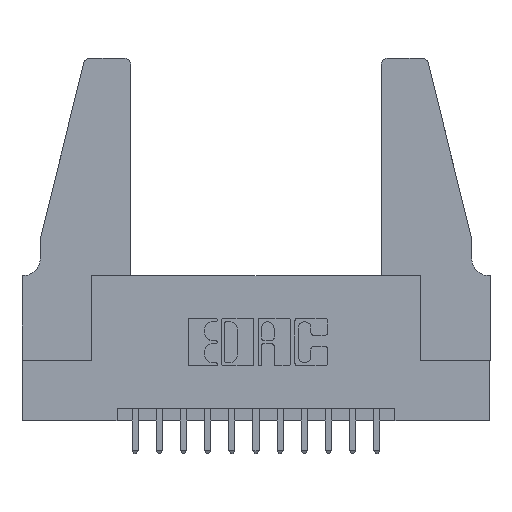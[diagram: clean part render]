
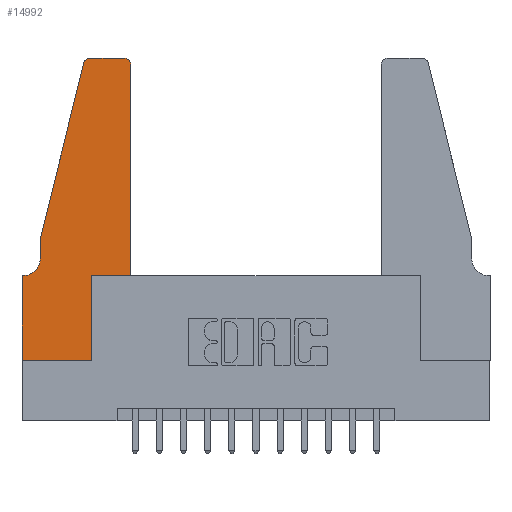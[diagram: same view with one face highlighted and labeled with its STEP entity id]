
A CAD part, top view. The second image highlights one B-rep face of the part: STEP entity #14992.
In plain terms, the highlighted planar face has unit normal (0, 0, 1).
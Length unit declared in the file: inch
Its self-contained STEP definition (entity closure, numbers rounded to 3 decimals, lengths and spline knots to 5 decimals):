
#108 = CARTESIAN_POINT ( 'NONE',  ( 0.0755, 0.5, 0.37 ) ) ;
#125 = VERTEX_POINT ( 'NONE', #3327 ) ;
#166 = DIRECTION ( 'NONE',  ( 0., -1., 0. ) ) ;
#212 = ORIENTED_EDGE ( 'NONE', *, *, #12947, .T. ) ;
#228 = EDGE_CURVE ( 'NONE', #125, #12000, #5634, .T. ) ;
#262 = CARTESIAN_POINT ( 'NONE',  ( 0.0755, 0.5, 0.37 ) ) ;
#379 = LINE ( 'NONE', #500, #3182 ) ;
#433 = CARTESIAN_POINT ( 'NONE',  ( 0.0755, 0.5, 0.37 ) ) ;
#470 = FACE_OUTER_BOUND ( 'NONE', #2129, .T. ) ;
#500 = CARTESIAN_POINT ( 'NONE',  ( 0., 0., 0.37 ) ) ;
#757 = EDGE_CURVE ( 'NONE', #13732, #3302, #10643, .T. ) ;
#803 = CARTESIAN_POINT ( 'NONE',  ( 0.284, 1.22, 0.37 ) ) ;
#858 = CARTESIAN_POINT ( 'NONE',  ( 0.284, 1.25, 0.37 ) ) ;
#1030 = VERTEX_POINT ( 'NONE', #3414 ) ;
#1486 = CIRCLE ( 'NONE', #11365, 0.03 ) ;
#1576 = VERTEX_POINT ( 'NONE', #4155 ) ;
#1954 = CARTESIAN_POINT ( 'NONE',  ( 0.2865, 0.35, 0.37 ) ) ;
#1992 = DIRECTION ( 'NONE',  ( 1., 0., 0. ) ) ;
#2028 = DIRECTION ( 'NONE',  ( 1., 0., 0. ) ) ;
#2129 = EDGE_LOOP ( 'NONE', ( #12750, #11359, #11556, #3574, #4023, #6680, #8276, #8024, #5431, #2158, #8148, #212 ) ) ;
#2158 = ORIENTED_EDGE ( 'NONE', *, *, #7189, .T. ) ;
#2525 = VECTOR ( 'NONE', #5208, 39.37008 ) ;
#2835 = LINE ( 'NONE', #433, #14681 ) ;
#2880 = EDGE_CURVE ( 'NONE', #14587, #1576, #11490, .T. ) ;
#2937 = CARTESIAN_POINT ( 'NONE',  ( 0.4505, 0.35, 0.37 ) ) ;
#2989 = EDGE_CURVE ( 'NONE', #12777, #125, #379, .T. ) ;
#3182 = VECTOR ( 'NONE', #9149, 39.37008 ) ;
#3302 = VERTEX_POINT ( 'NONE', #858 ) ;
#3327 = CARTESIAN_POINT ( 'NONE',  ( 0., 0., 0.37 ) ) ;
#3397 = CARTESIAN_POINT ( 'NONE',  ( 0., 0.35, 0.37 ) ) ;
#3414 = CARTESIAN_POINT ( 'NONE',  ( 0.4505, 1.22, 0.37 ) ) ;
#3507 = EDGE_CURVE ( 'NONE', #14669, #12777, #5528, .T. ) ;
#3574 = ORIENTED_EDGE ( 'NONE', *, *, #2880, .T. ) ;
#3804 = DIRECTION ( 'NONE',  ( 0., 0., -1. ) ) ;
#4023 = ORIENTED_EDGE ( 'NONE', *, *, #7883, .T. ) ;
#4064 = EDGE_CURVE ( 'NONE', #9768, #1030, #13223, .T. ) ;
#4136 = AXIS2_PLACEMENT_3D ( 'NONE', #803, #8943, #1992 ) ;
#4155 = CARTESIAN_POINT ( 'NONE',  ( 0.0755, 0.42, 0.37 ) ) ;
#4530 = VECTOR ( 'NONE', #4562, 39.37008 ) ;
#4562 = DIRECTION ( 'NONE',  ( -1., 0., 0. ) ) ;
#4564 = DIRECTION ( 'NONE',  ( 1., 0., 0. ) ) ;
#4651 = VECTOR ( 'NONE', #166, 39.37008 ) ;
#4653 = CARTESIAN_POINT ( 'NONE',  ( 0.4205, 1.25, 0.37 ) ) ;
#5072 = DIRECTION ( 'NONE',  ( 0., 0., 1. ) ) ;
#5208 = DIRECTION ( 'NONE',  ( 1., 0., 0. ) ) ;
#5271 = DIRECTION ( 'NONE',  ( 0., 1., 0. ) ) ;
#5431 = ORIENTED_EDGE ( 'NONE', *, *, #9946, .T. ) ;
#5528 = LINE ( 'NONE', #5904, #11278 ) ;
#5634 = LINE ( 'NONE', #11948, #2525 ) ;
#5657 = LINE ( 'NONE', #6684, #11762 ) ;
#5904 = CARTESIAN_POINT ( 'NONE',  ( 0.0755, 0.35, 0.37 ) ) ;
#6346 = DIRECTION ( 'NONE',  ( -0.239, -0.971, 0. ) ) ;
#6680 = ORIENTED_EDGE ( 'NONE', *, *, #3507, .T. ) ;
#6684 = CARTESIAN_POINT ( 'NONE',  ( 0.4505, 0.35, 0.37 ) ) ;
#7189 = EDGE_CURVE ( 'NONE', #9384, #9768, #5657, .T. ) ;
#7270 = AXIS2_PLACEMENT_3D ( 'NONE', #10701, #3804, #11851 ) ;
#7433 = CIRCLE ( 'NONE', #4136, 0.03 ) ;
#7443 = CARTESIAN_POINT ( 'NONE',  ( 0.0055, 0.35, 0.37 ) ) ;
#7883 = EDGE_CURVE ( 'NONE', #1576, #14669, #14197, .T. ) ;
#7901 = LINE ( 'NONE', #13316, #10595 ) ;
#8024 = ORIENTED_EDGE ( 'NONE', *, *, #228, .T. ) ;
#8148 = ORIENTED_EDGE ( 'NONE', *, *, #4064, .T. ) ;
#8276 = ORIENTED_EDGE ( 'NONE', *, *, #2989, .T. ) ;
#8448 = CARTESIAN_POINT ( 'NONE',  ( 0.4505, 0.35, 0.37 ) ) ;
#8943 = DIRECTION ( 'NONE',  ( 0., 0., 1. ) ) ;
#9149 = DIRECTION ( 'NONE',  ( 0., -1., 0. ) ) ;
#9369 = CARTESIAN_POINT ( 'NONE',  ( 0., 0.35, 0.37 ) ) ;
#9384 = VERTEX_POINT ( 'NONE', #1954 ) ;
#9768 = VERTEX_POINT ( 'NONE', #8448 ) ;
#9861 = EDGE_CURVE ( 'NONE', #11305, #14587, #2835, .T. ) ;
#9946 = EDGE_CURVE ( 'NONE', #12000, #9384, #7901, .T. ) ;
#10248 = PLANE ( 'NONE',  #13347 ) ;
#10595 = VECTOR ( 'NONE', #5271, 39.37008 ) ;
#10643 = LINE ( 'NONE', #10796, #4530 ) ;
#10701 = CARTESIAN_POINT ( 'NONE',  ( 0.0055, 0.42, 0.37 ) ) ;
#10796 = CARTESIAN_POINT ( 'NONE',  ( 0.2605, 1.25, 0.37 ) ) ;
#11278 = VECTOR ( 'NONE', #13663, 39.37008 ) ;
#11305 = VERTEX_POINT ( 'NONE', #13631 ) ;
#11359 = ORIENTED_EDGE ( 'NONE', *, *, #14873, .T. ) ;
#11365 = AXIS2_PLACEMENT_3D ( 'NONE', #11956, #5072, #13081 ) ;
#11457 = DIRECTION ( 'NONE',  ( 0., 0., 1. ) ) ;
#11490 = LINE ( 'NONE', #108, #4651 ) ;
#11555 = DIRECTION ( 'NONE',  ( 0., 1., 0. ) ) ;
#11556 = ORIENTED_EDGE ( 'NONE', *, *, #9861, .T. ) ;
#11762 = VECTOR ( 'NONE', #2028, 39.37008 ) ;
#11851 = DIRECTION ( 'NONE',  ( -1., 0., 0. ) ) ;
#11948 = CARTESIAN_POINT ( 'NONE',  ( 0., 0., 0.37 ) ) ;
#11956 = CARTESIAN_POINT ( 'NONE',  ( 0.4205, 1.22, 0.37 ) ) ;
#12000 = VERTEX_POINT ( 'NONE', #13704 ) ;
#12750 = ORIENTED_EDGE ( 'NONE', *, *, #757, .T. ) ;
#12777 = VERTEX_POINT ( 'NONE', #9369 ) ;
#12947 = EDGE_CURVE ( 'NONE', #1030, #13732, #1486, .T. ) ;
#13081 = DIRECTION ( 'NONE',  ( 1., 0., 0. ) ) ;
#13223 = LINE ( 'NONE', #2937, #13586 ) ;
#13316 = CARTESIAN_POINT ( 'NONE',  ( 0.2865, 0.35, 0.37 ) ) ;
#13347 = AXIS2_PLACEMENT_3D ( 'NONE', #3397, #11457, #4564 ) ;
#13586 = VECTOR ( 'NONE', #11555, 39.37008 ) ;
#13631 = CARTESIAN_POINT ( 'NONE',  ( 0.25487, 1.22718, 0.37 ) ) ;
#13663 = DIRECTION ( 'NONE',  ( -1., 0., 0. ) ) ;
#13704 = CARTESIAN_POINT ( 'NONE',  ( 0.2865, 0., 0.37 ) ) ;
#13732 = VERTEX_POINT ( 'NONE', #4653 ) ;
#14197 = CIRCLE ( 'NONE', #7270, 0.07 ) ;
#14587 = VERTEX_POINT ( 'NONE', #262 ) ;
#14669 = VERTEX_POINT ( 'NONE', #7443 ) ;
#14681 = VECTOR ( 'NONE', #6346, 39.37008 ) ;
#14873 = EDGE_CURVE ( 'NONE', #3302, #11305, #7433, .T. ) ;
#14992 = ADVANCED_FACE ( 'NONE', ( #470 ), #10248, .T. ) ;
